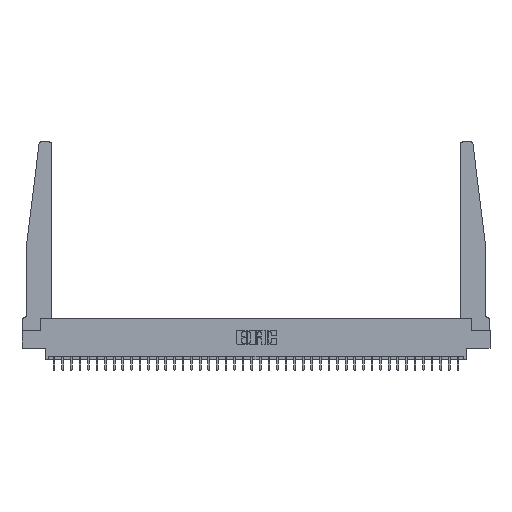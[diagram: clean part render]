
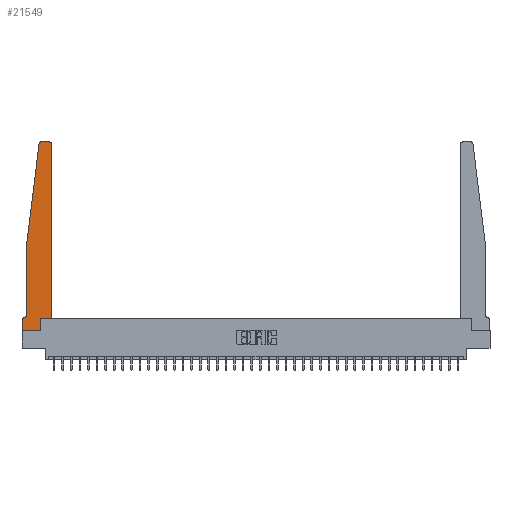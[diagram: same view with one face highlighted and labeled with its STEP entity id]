
A CAD part, top view. The second image highlights one B-rep face of the part: STEP entity #21549.
In plain terms, the highlighted planar face has unit normal (0, 0, 1).
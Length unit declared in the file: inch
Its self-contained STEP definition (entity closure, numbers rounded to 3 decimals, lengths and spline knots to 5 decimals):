
#562 = VECTOR ( 'NONE', #4618, 39.37008 ) ;
#567 = ORIENTED_EDGE ( 'NONE', *, *, #1256, .T. ) ;
#770 = VERTEX_POINT ( 'NONE', #23567 ) ;
#1256 = EDGE_CURVE ( 'NONE', #24451, #12226, #14217, .T. ) ;
#1310 = EDGE_CURVE ( 'NONE', #19467, #9153, #10086, .T. ) ;
#1341 = CARTESIAN_POINT ( 'NONE',  ( 0., 0.1875, 0.37 ) ) ;
#1355 = DIRECTION ( 'NONE',  ( 1., 0., 0. ) ) ;
#1654 = DIRECTION ( 'NONE',  ( -1., 0., 0. ) ) ;
#1680 = CIRCLE ( 'NONE', #26639, 0.03 ) ;
#2635 = VERTEX_POINT ( 'NONE', #11194 ) ;
#2895 = VERTEX_POINT ( 'NONE', #26058 ) ;
#2913 = VECTOR ( 'NONE', #1654, 39.37008 ) ;
#3822 = ORIENTED_EDGE ( 'NONE', *, *, #18545, .T. ) ;
#4057 = DIRECTION ( 'NONE',  ( 1., 0., 0. ) ) ;
#4273 = CARTESIAN_POINT ( 'NONE',  ( 0.065, 1.25, 0.37 ) ) ;
#4293 = DIRECTION ( 'NONE',  ( 0., -1., 0. ) ) ;
#4618 = DIRECTION ( 'NONE',  ( 0., 1., 0. ) ) ;
#5604 = EDGE_CURVE ( 'NONE', #2895, #29923, #11564, .T. ) ;
#5966 = DIRECTION ( 'NONE',  ( -1., 0., 0. ) ) ;
#6504 = VECTOR ( 'NONE', #32506, 39.37008 ) ;
#6819 = AXIS2_PLACEMENT_3D ( 'NONE', #18328, #24331, #27226 ) ;
#7335 = CARTESIAN_POINT ( 'NONE',  ( 0.27653, 2.75, 0.37 ) ) ;
#7380 = LINE ( 'NONE', #12847, #20611 ) ;
#9153 = VERTEX_POINT ( 'NONE', #22392 ) ;
#9590 = VERTEX_POINT ( 'NONE', #28328 ) ;
#9615 = ORIENTED_EDGE ( 'NONE', *, *, #12734, .T. ) ;
#10064 = CARTESIAN_POINT ( 'NONE',  ( 0.395, 2.75, 0.37 ) ) ;
#10086 = LINE ( 'NONE', #4273, #20927 ) ;
#10195 = LINE ( 'NONE', #12566, #27002 ) ;
#10269 = CARTESIAN_POINT ( 'NONE',  ( 0.395, 2.72, 0.37 ) ) ;
#10663 = LINE ( 'NONE', #21739, #15831 ) ;
#10835 = CARTESIAN_POINT ( 'NONE',  ( 0.27653, 2.72, 0.37 ) ) ;
#11194 = CARTESIAN_POINT ( 'NONE',  ( 0.2605, 0., 0.37 ) ) ;
#11564 = CIRCLE ( 'NONE', #28952, 0.05 ) ;
#11783 = DIRECTION ( 'NONE',  ( 0., 0., -1. ) ) ;
#12201 = EDGE_CURVE ( 'NONE', #9590, #24451, #14809, .T. ) ;
#12226 = VERTEX_POINT ( 'NONE', #10064 ) ;
#12444 = VECTOR ( 'NONE', #34412, 39.37008 ) ;
#12532 = CARTESIAN_POINT ( 'NONE',  ( 0.2605, 0.18, 0.37 ) ) ;
#12566 = CARTESIAN_POINT ( 'NONE',  ( 0.2605, 0.18, 0.37 ) ) ;
#12734 = EDGE_CURVE ( 'NONE', #12226, #32237, #26541, .T. ) ;
#12847 = CARTESIAN_POINT ( 'NONE',  ( 0.065, 1.25, 0.37 ) ) ;
#13252 = PLANE ( 'NONE',  #6819 ) ;
#13443 = LINE ( 'NONE', #32855, #6504 ) ;
#13493 = VECTOR ( 'NONE', #4057, 39.37008 ) ;
#13970 = ORIENTED_EDGE ( 'NONE', *, *, #1310, .T. ) ;
#14217 = CIRCLE ( 'NONE', #34491, 0.03 ) ;
#14404 = ORIENTED_EDGE ( 'NONE', *, *, #16539, .T. ) ;
#14618 = EDGE_LOOP ( 'NONE', ( #9615, #22755, #13970, #24891, #34543, #14404, #20374, #3822, #14923, #33101, #21071, #567 ) ) ;
#14809 = LINE ( 'NONE', #26231, #562 ) ;
#14834 = CARTESIAN_POINT ( 'NONE',  ( 0.24675, 2.72367, 0.37 ) ) ;
#14923 = ORIENTED_EDGE ( 'NONE', *, *, #28830, .T. ) ;
#15348 = LINE ( 'NONE', #25865, #12444 ) ;
#15370 = DIRECTION ( 'NONE',  ( -0.122, -0.992, 0. ) ) ;
#15831 = VECTOR ( 'NONE', #32814, 39.37008 ) ;
#15939 = EDGE_CURVE ( 'NONE', #22361, #770, #13443, .T. ) ;
#16539 = EDGE_CURVE ( 'NONE', #29923, #22361, #10663, .T. ) ;
#17516 = CARTESIAN_POINT ( 'NONE',  ( 0., 0., 0.37 ) ) ;
#17867 = LINE ( 'NONE', #17516, #13493 ) ;
#18328 = CARTESIAN_POINT ( 'NONE',  ( 0., 0.1875, 0.37 ) ) ;
#18456 = DIRECTION ( 'NONE',  ( 0., 0., 1. ) ) ;
#18545 = EDGE_CURVE ( 'NONE', #770, #2635, #17867, .T. ) ;
#19467 = VERTEX_POINT ( 'NONE', #14834 ) ;
#20374 = ORIENTED_EDGE ( 'NONE', *, *, #15939, .T. ) ;
#20611 = VECTOR ( 'NONE', #4293, 39.37008 ) ;
#20927 = VECTOR ( 'NONE', #15370, 39.37008 ) ;
#21071 = ORIENTED_EDGE ( 'NONE', *, *, #12201, .T. ) ;
#21549 = ADVANCED_FACE ( 'NONE', ( #26493 ), #13252, .T. ) ;
#21739 = CARTESIAN_POINT ( 'NONE',  ( 0.065, 0.1875, 0.37 ) ) ;
#21916 = DIRECTION ( 'NONE',  ( 0., 0., 1. ) ) ;
#22361 = VERTEX_POINT ( 'NONE', #1341 ) ;
#22392 = CARTESIAN_POINT ( 'NONE',  ( 0.065, 1.25, 0.37 ) ) ;
#22508 = CARTESIAN_POINT ( 'NONE',  ( 0.015, 0.2375, 0.37 ) ) ;
#22755 = ORIENTED_EDGE ( 'NONE', *, *, #23314, .T. ) ;
#23314 = EDGE_CURVE ( 'NONE', #32237, #19467, #1680, .T. ) ;
#23567 = CARTESIAN_POINT ( 'NONE',  ( 0., 0., 0.37 ) ) ;
#23825 = CARTESIAN_POINT ( 'NONE',  ( 0.25, 2.75, 0.37 ) ) ;
#24331 = DIRECTION ( 'NONE',  ( 0., 0., 1. ) ) ;
#24451 = VERTEX_POINT ( 'NONE', #33916 ) ;
#24764 = CARTESIAN_POINT ( 'NONE',  ( 0.015, 0.1875, 0.37 ) ) ;
#24891 = ORIENTED_EDGE ( 'NONE', *, *, #27052, .T. ) ;
#25865 = CARTESIAN_POINT ( 'NONE',  ( 0.425, 0.18, 0.37 ) ) ;
#26058 = CARTESIAN_POINT ( 'NONE',  ( 0.065, 0.2375, 0.37 ) ) ;
#26231 = CARTESIAN_POINT ( 'NONE',  ( 0.425, 0.18, 0.37 ) ) ;
#26330 = EDGE_CURVE ( 'NONE', #34352, #9590, #15348, .T. ) ;
#26493 = FACE_OUTER_BOUND ( 'NONE', #14618, .T. ) ;
#26541 = LINE ( 'NONE', #23825, #2913 ) ;
#26639 = AXIS2_PLACEMENT_3D ( 'NONE', #10835, #21916, #27717 ) ;
#27002 = VECTOR ( 'NONE', #34734, 39.37008 ) ;
#27052 = EDGE_CURVE ( 'NONE', #9153, #2895, #7380, .T. ) ;
#27226 = DIRECTION ( 'NONE',  ( 1., 0., 0. ) ) ;
#27717 = DIRECTION ( 'NONE',  ( 1., 0., 0. ) ) ;
#28328 = CARTESIAN_POINT ( 'NONE',  ( 0.425, 0.18, 0.37 ) ) ;
#28830 = EDGE_CURVE ( 'NONE', #2635, #34352, #10195, .T. ) ;
#28952 = AXIS2_PLACEMENT_3D ( 'NONE', #22508, #11783, #5966 ) ;
#29923 = VERTEX_POINT ( 'NONE', #24764 ) ;
#32237 = VERTEX_POINT ( 'NONE', #7335 ) ;
#32506 = DIRECTION ( 'NONE',  ( 0., -1., 0. ) ) ;
#32814 = DIRECTION ( 'NONE',  ( -1., 0., 0. ) ) ;
#32855 = CARTESIAN_POINT ( 'NONE',  ( 0., 0., 0.37 ) ) ;
#33101 = ORIENTED_EDGE ( 'NONE', *, *, #26330, .T. ) ;
#33916 = CARTESIAN_POINT ( 'NONE',  ( 0.425, 2.72, 0.37 ) ) ;
#34352 = VERTEX_POINT ( 'NONE', #12532 ) ;
#34412 = DIRECTION ( 'NONE',  ( 1., 0., 0. ) ) ;
#34491 = AXIS2_PLACEMENT_3D ( 'NONE', #10269, #18456, #1355 ) ;
#34543 = ORIENTED_EDGE ( 'NONE', *, *, #5604, .T. ) ;
#34734 = DIRECTION ( 'NONE',  ( 0., 1., 0. ) ) ;
